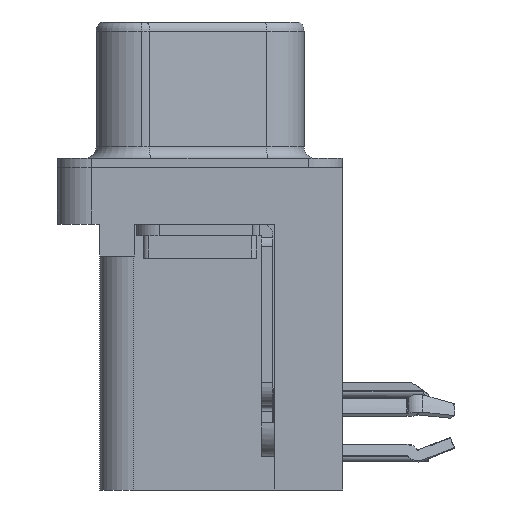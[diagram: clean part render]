
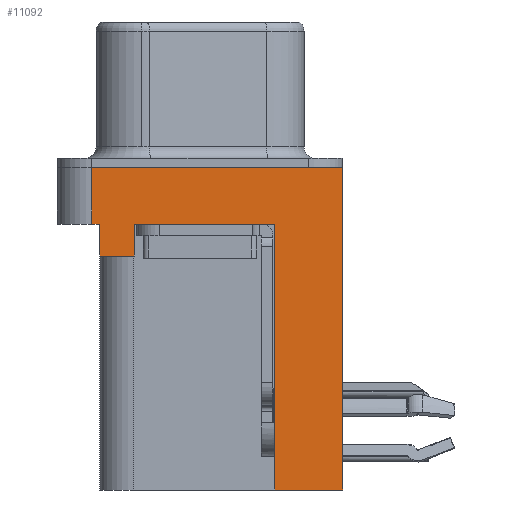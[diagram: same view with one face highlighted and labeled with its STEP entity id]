
A CAD part, left-side view. The second image highlights one B-rep face of the part: STEP entity #11092.
In plain terms, the highlighted planar face has unit normal (-1, 0, 0).
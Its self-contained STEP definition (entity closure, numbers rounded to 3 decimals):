
#100 = DIRECTION ( 'NONE',  ( 0., 1., 0. ) ) ;
#522 = CARTESIAN_POINT ( 'NONE',  ( -2.91, 2.895, -3.9 ) ) ;
#711 = DIRECTION ( 'NONE',  ( 0., -1., 0. ) ) ;
#1225 = DIRECTION ( 'NONE',  ( 0., -1., 0. ) ) ;
#1516 = FACE_OUTER_BOUND ( 'NONE', #23021, .T. ) ;
#1597 = CARTESIAN_POINT ( 'NONE',  ( -2.91, 4.425, -3.9 ) ) ;
#1647 = CARTESIAN_POINT ( 'NONE',  ( -2.91, -6.275, -2.5 ) ) ;
#1846 = VERTEX_POINT ( 'NONE', #24301 ) ;
#2652 = VERTEX_POINT ( 'NONE', #17498 ) ;
#2736 = VERTEX_POINT ( 'NONE', #10308 ) ;
#3247 = LINE ( 'NONE', #16112, #11717 ) ;
#3306 = VECTOR ( 'NONE', #100, 1000. ) ;
#4354 = VERTEX_POINT ( 'NONE', #18988 ) ;
#4729 = DIRECTION ( 'NONE',  ( 0., 0., 1. ) ) ;
#5090 = CARTESIAN_POINT ( 'NONE',  ( -2.91, -6.275, -2.5 ) ) ;
#5125 = ORIENTED_EDGE ( 'NONE', *, *, #19281, .T. ) ;
#5384 = DIRECTION ( 'NONE',  ( -1., 0., 0. ) ) ;
#5587 = VECTOR ( 'NONE', #24156, 1000. ) ;
#5848 = LINE ( 'NONE', #9976, #3306 ) ;
#5855 = LINE ( 'NONE', #22422, #12151 ) ;
#6051 = EDGE_CURVE ( 'NONE', #22239, #24140, #5855, .T. ) ;
#6293 = VERTEX_POINT ( 'NONE', #11297 ) ;
#6307 = VECTOR ( 'NONE', #1225, 1000. ) ;
#6450 = LINE ( 'NONE', #10840, #10251 ) ;
#7579 = ORIENTED_EDGE ( 'NONE', *, *, #10056, .F. ) ;
#7636 = DIRECTION ( 'NONE',  ( 0., -1., 0. ) ) ;
#7780 = EDGE_CURVE ( 'NONE', #4354, #6293, #15908, .T. ) ;
#7996 = DIRECTION ( 'NONE',  ( 0., 0., 1. ) ) ;
#8401 = EDGE_CURVE ( 'NONE', #1846, #2652, #15314, .T. ) ;
#8801 = ORIENTED_EDGE ( 'NONE', *, *, #6051, .F. ) ;
#8977 = VECTOR ( 'NONE', #7996, 1000. ) ;
#9232 = VERTEX_POINT ( 'NONE', #16557 ) ;
#9860 = LINE ( 'NONE', #20183, #8977 ) ;
#9976 = CARTESIAN_POINT ( 'NONE',  ( -2.91, -3.295, -14.2 ) ) ;
#10056 = EDGE_CURVE ( 'NONE', #1846, #9232, #15716, .T. ) ;
#10251 = VECTOR ( 'NONE', #711, 1000. ) ;
#10308 = CARTESIAN_POINT ( 'NONE',  ( -2.91, 2.895, -2.5 ) ) ;
#10840 = CARTESIAN_POINT ( 'NONE',  ( -2.91, -6.275, 0. ) ) ;
#10942 = ORIENTED_EDGE ( 'NONE', *, *, #13641, .F. ) ;
#11092 = ADVANCED_FACE ( 'NONE', ( #1516 ), #11764, .T. ) ;
#11297 = CARTESIAN_POINT ( 'NONE',  ( -2.91, -6.275, 0. ) ) ;
#11311 = CARTESIAN_POINT ( 'NONE',  ( -2.91, -3.295, -2.5 ) ) ;
#11717 = VECTOR ( 'NONE', #7636, 1000. ) ;
#11764 = PLANE ( 'NONE',  #24990 ) ;
#11972 = DIRECTION ( 'NONE',  ( 0., 1., 0. ) ) ;
#12151 = VECTOR ( 'NONE', #11972, 1000. ) ;
#12731 = VERTEX_POINT ( 'NONE', #19984 ) ;
#12924 = EDGE_CURVE ( 'NONE', #9232, #6293, #6450, .T. ) ;
#13369 = ORIENTED_EDGE ( 'NONE', *, *, #12924, .F. ) ;
#13489 = DIRECTION ( 'NONE',  ( 0., 0., 1. ) ) ;
#13641 = EDGE_CURVE ( 'NONE', #24140, #2652, #21642, .T. ) ;
#14247 = ORIENTED_EDGE ( 'NONE', *, *, #20548, .T. ) ;
#14535 = ORIENTED_EDGE ( 'NONE', *, *, #23780, .F. ) ;
#14759 = VECTOR ( 'NONE', #4729, 1000. ) ;
#14872 = EDGE_CURVE ( 'NONE', #12731, #18606, #9860, .T. ) ;
#15314 = LINE ( 'NONE', #5090, #6307 ) ;
#15584 = DIRECTION ( 'NONE',  ( 0., 0., 1. ) ) ;
#15716 = LINE ( 'NONE', #19822, #20704 ) ;
#15908 = LINE ( 'NONE', #18275, #14759 ) ;
#15961 = CARTESIAN_POINT ( 'NONE',  ( -2.91, 2.895, -3.9 ) ) ;
#16112 = CARTESIAN_POINT ( 'NONE',  ( -2.91, -6.275, -2.5 ) ) ;
#16557 = CARTESIAN_POINT ( 'NONE',  ( -2.91, 4.775, 0. ) ) ;
#17498 = CARTESIAN_POINT ( 'NONE',  ( -2.91, 4.425, -2.5 ) ) ;
#18275 = CARTESIAN_POINT ( 'NONE',  ( -2.91, -6.275, -2.5 ) ) ;
#18606 = VERTEX_POINT ( 'NONE', #11311 ) ;
#18750 = ORIENTED_EDGE ( 'NONE', *, *, #8401, .T. ) ;
#18835 = VECTOR ( 'NONE', #22562, 1000. ) ;
#18988 = CARTESIAN_POINT ( 'NONE',  ( -2.91, -6.275, -14.2 ) ) ;
#19281 = EDGE_CURVE ( 'NONE', #22239, #2736, #24558, .T. ) ;
#19822 = CARTESIAN_POINT ( 'NONE',  ( -2.91, 4.775, -2.5 ) ) ;
#19984 = CARTESIAN_POINT ( 'NONE',  ( -2.91, -3.295, -14.2 ) ) ;
#20183 = CARTESIAN_POINT ( 'NONE',  ( -2.91, -3.295, -14.2 ) ) ;
#20548 = EDGE_CURVE ( 'NONE', #2736, #18606, #3247, .T. ) ;
#20704 = VECTOR ( 'NONE', #15584, 1000. ) ;
#21642 = LINE ( 'NONE', #1597, #5587 ) ;
#22239 = VERTEX_POINT ( 'NONE', #15961 ) ;
#22422 = CARTESIAN_POINT ( 'NONE',  ( -2.91, 4.425, -3.9 ) ) ;
#22562 = DIRECTION ( 'NONE',  ( 0., 0., 1. ) ) ;
#22777 = ORIENTED_EDGE ( 'NONE', *, *, #7780, .T. ) ;
#23021 = EDGE_LOOP ( 'NONE', ( #13369, #7579, #18750, #10942, #8801, #5125, #14247, #23535, #14535, #22777 ) ) ;
#23535 = ORIENTED_EDGE ( 'NONE', *, *, #14872, .F. ) ;
#23780 = EDGE_CURVE ( 'NONE', #4354, #12731, #5848, .T. ) ;
#24140 = VERTEX_POINT ( 'NONE', #24483 ) ;
#24156 = DIRECTION ( 'NONE',  ( 0., 0., 1. ) ) ;
#24301 = CARTESIAN_POINT ( 'NONE',  ( -2.91, 4.775, -2.5 ) ) ;
#24483 = CARTESIAN_POINT ( 'NONE',  ( -2.91, 4.425, -3.9 ) ) ;
#24558 = LINE ( 'NONE', #522, #18835 ) ;
#24990 = AXIS2_PLACEMENT_3D ( 'NONE', #1647, #5384, #13489 ) ;
